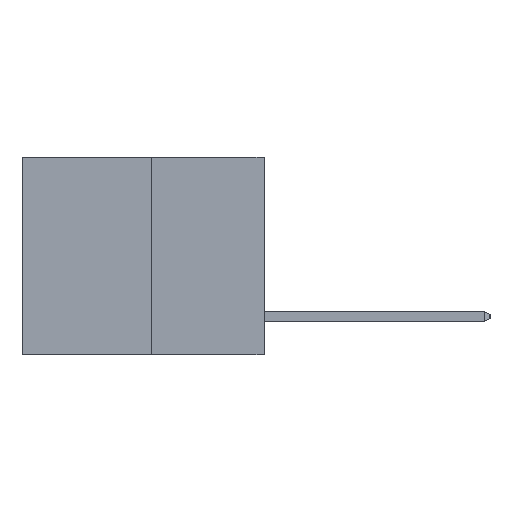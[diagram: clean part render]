
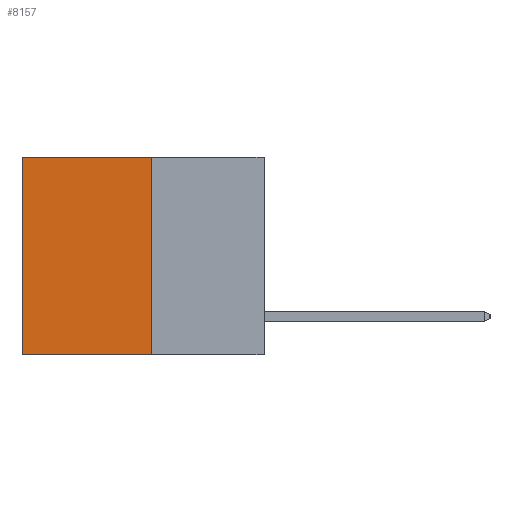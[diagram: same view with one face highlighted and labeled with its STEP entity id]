
A CAD part, left-side view. The second image highlights one B-rep face of the part: STEP entity #8157.
In plain terms, the highlighted planar face has unit normal (-1, 0, 0).
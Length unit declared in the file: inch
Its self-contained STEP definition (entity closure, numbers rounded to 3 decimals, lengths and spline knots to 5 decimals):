
#912 = CARTESIAN_POINT ( 'NONE',  ( 0.3165, 0.28, 0. ) ) ;
#1046 = VERTEX_POINT ( 'NONE', #20237 ) ;
#2337 = VECTOR ( 'NONE', #7583, 39.37008 ) ;
#2405 = EDGE_LOOP ( 'NONE', ( #5041, #20396, #22035, #17426 ) ) ;
#3397 = CARTESIAN_POINT ( 'NONE',  ( 0.3165, 0.28, -0.49 ) ) ;
#3487 = DIRECTION ( 'NONE',  ( 0., 0., -1. ) ) ;
#3927 = VERTEX_POINT ( 'NONE', #7373 ) ;
#4394 = CARTESIAN_POINT ( 'NONE',  ( 0.3165, 0.6, -0.49 ) ) ;
#5041 = ORIENTED_EDGE ( 'NONE', *, *, #7038, .T. ) ;
#5900 = LINE ( 'NONE', #912, #20288 ) ;
#6666 = VERTEX_POINT ( 'NONE', #18548 ) ;
#7038 = EDGE_CURVE ( 'NONE', #1046, #3927, #18661, .T. ) ;
#7162 = VECTOR ( 'NONE', #3487, 39.37008 ) ;
#7204 = EDGE_CURVE ( 'NONE', #6666, #1046, #5900, .T. ) ;
#7373 = CARTESIAN_POINT ( 'NONE',  ( 0.3165, 0.6, -0.49 ) ) ;
#7583 = DIRECTION ( 'NONE',  ( 0., 1., 0. ) ) ;
#8157 = ADVANCED_FACE ( 'NONE', ( #15787 ), #22715, .F. ) ;
#9323 = CARTESIAN_POINT ( 'NONE',  ( 0.3165, 0.28, -0.49 ) ) ;
#9628 = EDGE_CURVE ( 'NONE', #6666, #15305, #16580, .T. ) ;
#11569 = DIRECTION ( 'NONE',  ( 0., 1., 0. ) ) ;
#12248 = LINE ( 'NONE', #9323, #2337 ) ;
#12394 = DIRECTION ( 'NONE',  ( 0., 0., -1. ) ) ;
#13856 = CARTESIAN_POINT ( 'NONE',  ( 0.3165, 0.28, -0.49 ) ) ;
#14735 = VECTOR ( 'NONE', #19117, 39.37008 ) ;
#15305 = VERTEX_POINT ( 'NONE', #19020 ) ;
#15787 = FACE_OUTER_BOUND ( 'NONE', #2405, .T. ) ;
#16580 = LINE ( 'NONE', #3397, #7162 ) ;
#17423 = DIRECTION ( 'NONE',  ( 1., 0., 0. ) ) ;
#17426 = ORIENTED_EDGE ( 'NONE', *, *, #7204, .T. ) ;
#18548 = CARTESIAN_POINT ( 'NONE',  ( 0.3165, 0.28, 0. ) ) ;
#18661 = LINE ( 'NONE', #4394, #14735 ) ;
#19020 = CARTESIAN_POINT ( 'NONE',  ( 0.3165, 0.28, -0.49 ) ) ;
#19117 = DIRECTION ( 'NONE',  ( 0., 0., -1. ) ) ;
#20237 = CARTESIAN_POINT ( 'NONE',  ( 0.3165, 0.6, 0. ) ) ;
#20288 = VECTOR ( 'NONE', #11569, 39.37008 ) ;
#20396 = ORIENTED_EDGE ( 'NONE', *, *, #20945, .F. ) ;
#20911 = AXIS2_PLACEMENT_3D ( 'NONE', #13856, #17423, #12394 ) ;
#20945 = EDGE_CURVE ( 'NONE', #15305, #3927, #12248, .T. ) ;
#22035 = ORIENTED_EDGE ( 'NONE', *, *, #9628, .F. ) ;
#22715 = PLANE ( 'NONE',  #20911 ) ;
